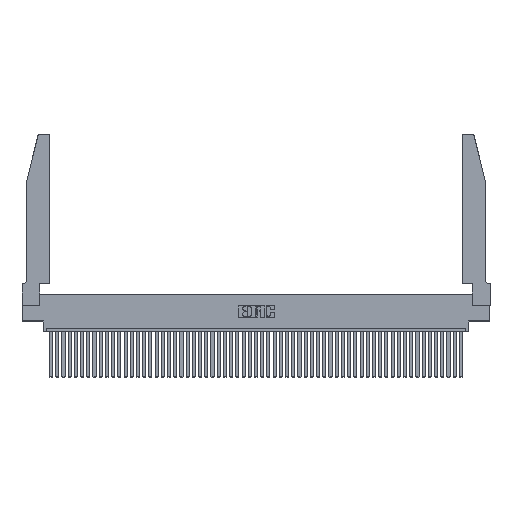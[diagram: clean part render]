
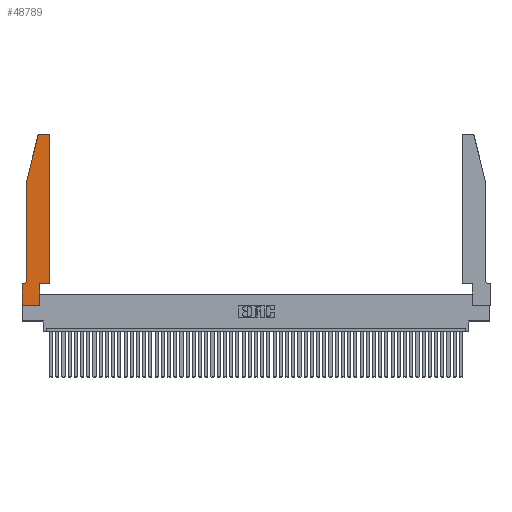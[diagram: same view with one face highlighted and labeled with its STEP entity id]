
A CAD part, top view. The second image highlights one B-rep face of the part: STEP entity #48789.
In plain terms, the highlighted planar face has unit normal (0, 0, 1).
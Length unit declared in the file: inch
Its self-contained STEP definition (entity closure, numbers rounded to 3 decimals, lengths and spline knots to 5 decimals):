
#66 = EDGE_CURVE ( 'NONE', #10024, #24313, #39739, .T. ) ;
#1700 = CARTESIAN_POINT ( 'NONE',  ( 0.2865, 0.35, 0.37 ) ) ;
#1920 = CARTESIAN_POINT ( 'NONE',  ( 0.2865, 0., 0.37 ) ) ;
#2434 = CARTESIAN_POINT ( 'NONE',  ( 0., 0., 0.37 ) ) ;
#2527 = VERTEX_POINT ( 'NONE', #1920 ) ;
#2875 = VECTOR ( 'NONE', #14905, 39.37008 ) ;
#3215 = EDGE_LOOP ( 'NONE', ( #14793, #34141, #24179, #48476, #18701, #36533, #26849, #27975, #34392, #27274, #50591, #46107 ) ) ;
#4255 = LINE ( 'NONE', #2434, #35532 ) ;
#4756 = VERTEX_POINT ( 'NONE', #42037 ) ;
#4902 = DIRECTION ( 'NONE',  ( 1., 0., 0. ) ) ;
#5426 = EDGE_CURVE ( 'NONE', #31566, #41945, #10612, .T. ) ;
#5642 = CARTESIAN_POINT ( 'NONE',  ( 0.284, 2.75, 0.37 ) ) ;
#7010 = CARTESIAN_POINT ( 'NONE',  ( 0.4205, 2.75, 0.37 ) ) ;
#7765 = DIRECTION ( 'NONE',  ( 0., 1., 0. ) ) ;
#8401 = LINE ( 'NONE', #18358, #28342 ) ;
#8618 = EDGE_CURVE ( 'NONE', #25354, #40194, #20551, .T. ) ;
#9263 = CARTESIAN_POINT ( 'NONE',  ( 0.0055, 0.42, 0.37 ) ) ;
#9737 = LINE ( 'NONE', #40828, #10432 ) ;
#10024 = VERTEX_POINT ( 'NONE', #45521 ) ;
#10281 = EDGE_CURVE ( 'NONE', #51760, #2527, #4255, .T. ) ;
#10432 = VECTOR ( 'NONE', #12880, 39.37008 ) ;
#10612 = LINE ( 'NONE', #22920, #39987 ) ;
#11596 = CARTESIAN_POINT ( 'NONE',  ( 0.4505, 0.35, 0.37 ) ) ;
#12880 = DIRECTION ( 'NONE',  ( -1., 0., 0. ) ) ;
#12923 = VECTOR ( 'NONE', #15116, 39.37008 ) ;
#13255 = DIRECTION ( 'NONE',  ( 0., 0., -1. ) ) ;
#13707 = VERTEX_POINT ( 'NONE', #30761 ) ;
#14534 = EDGE_CURVE ( 'NONE', #41945, #25354, #19542, .T. ) ;
#14793 = ORIENTED_EDGE ( 'NONE', *, *, #22210, .T. ) ;
#14905 = DIRECTION ( 'NONE',  ( -0.239, -0.971, 0. ) ) ;
#15116 = DIRECTION ( 'NONE',  ( 0., -1., 0. ) ) ;
#15321 = AXIS2_PLACEMENT_3D ( 'NONE', #49514, #17477, #21470 ) ;
#15543 = DIRECTION ( 'NONE',  ( 0., -1., 0. ) ) ;
#16575 = EDGE_CURVE ( 'NONE', #2527, #31566, #41148, .T. ) ;
#17477 = DIRECTION ( 'NONE',  ( 0., 0., 1. ) ) ;
#17835 = PLANE ( 'NONE',  #15321 ) ;
#18030 = CARTESIAN_POINT ( 'NONE',  ( 0., 0.35, 0.37 ) ) ;
#18358 = CARTESIAN_POINT ( 'NONE',  ( 0.2605, 2.75, 0.37 ) ) ;
#18701 = ORIENTED_EDGE ( 'NONE', *, *, #32629, .T. ) ;
#18705 = CARTESIAN_POINT ( 'NONE',  ( 0.0755, 2., 0.37 ) ) ;
#18867 = CARTESIAN_POINT ( 'NONE',  ( 0., 0., 0.37 ) ) ;
#19542 = LINE ( 'NONE', #11596, #29456 ) ;
#20551 = CIRCLE ( 'NONE', #43430, 0.03 ) ;
#20673 = CARTESIAN_POINT ( 'NONE',  ( 0.2865, 0.35, 0.37 ) ) ;
#20701 = CARTESIAN_POINT ( 'NONE',  ( 0.4205, 2.72, 0.37 ) ) ;
#21470 = DIRECTION ( 'NONE',  ( 1., 0., 0. ) ) ;
#22210 = EDGE_CURVE ( 'NONE', #40194, #28152, #8401, .T. ) ;
#22470 = DIRECTION ( 'NONE',  ( 1., 0., 0. ) ) ;
#22606 = CARTESIAN_POINT ( 'NONE',  ( 0.0755, 2., 0.37 ) ) ;
#22920 = CARTESIAN_POINT ( 'NONE',  ( 0.4505, 0.35, 0.37 ) ) ;
#22939 = LINE ( 'NONE', #22606, #12923 ) ;
#24179 = ORIENTED_EDGE ( 'NONE', *, *, #66, .T. ) ;
#24313 = VERTEX_POINT ( 'NONE', #28280 ) ;
#25354 = VERTEX_POINT ( 'NONE', #32321 ) ;
#26849 = ORIENTED_EDGE ( 'NONE', *, *, #44274, .T. ) ;
#26972 = DIRECTION ( 'NONE',  ( 1., 0., 0. ) ) ;
#27183 = FACE_OUTER_BOUND ( 'NONE', #3215, .T. ) ;
#27274 = ORIENTED_EDGE ( 'NONE', *, *, #5426, .T. ) ;
#27350 = DIRECTION ( 'NONE',  ( -1., 0., 0. ) ) ;
#27456 = CARTESIAN_POINT ( 'NONE',  ( 0., 0., 0.37 ) ) ;
#27975 = ORIENTED_EDGE ( 'NONE', *, *, #10281, .T. ) ;
#28152 = VERTEX_POINT ( 'NONE', #5642 ) ;
#28280 = CARTESIAN_POINT ( 'NONE',  ( 0.0755, 2., 0.37 ) ) ;
#28342 = VECTOR ( 'NONE', #27350, 39.37008 ) ;
#29274 = DIRECTION ( 'NONE',  ( -1., 0., 0. ) ) ;
#29456 = VECTOR ( 'NONE', #7765, 39.37008 ) ;
#30566 = VECTOR ( 'NONE', #44882, 39.37008 ) ;
#30761 = CARTESIAN_POINT ( 'NONE',  ( 0.0055, 0.35, 0.37 ) ) ;
#31566 = VERTEX_POINT ( 'NONE', #1700 ) ;
#31842 = CARTESIAN_POINT ( 'NONE',  ( 0.4505, 0.35, 0.37 ) ) ;
#32321 = CARTESIAN_POINT ( 'NONE',  ( 0.4505, 2.72, 0.37 ) ) ;
#32629 = EDGE_CURVE ( 'NONE', #4756, #13707, #36383, .T. ) ;
#33253 = AXIS2_PLACEMENT_3D ( 'NONE', #9263, #13255, #29274 ) ;
#34141 = ORIENTED_EDGE ( 'NONE', *, *, #34300, .T. ) ;
#34300 = EDGE_CURVE ( 'NONE', #28152, #10024, #47662, .T. ) ;
#34392 = ORIENTED_EDGE ( 'NONE', *, *, #16575, .T. ) ;
#34593 = VERTEX_POINT ( 'NONE', #18030 ) ;
#35532 = VECTOR ( 'NONE', #22470, 39.37008 ) ;
#36383 = CIRCLE ( 'NONE', #33253, 0.07 ) ;
#36533 = ORIENTED_EDGE ( 'NONE', *, *, #39883, .T. ) ;
#37733 = CARTESIAN_POINT ( 'NONE',  ( 0.284, 2.72, 0.37 ) ) ;
#39380 = VECTOR ( 'NONE', #15543, 39.37008 ) ;
#39534 = DIRECTION ( 'NONE',  ( 0., 0., 1. ) ) ;
#39739 = LINE ( 'NONE', #18705, #2875 ) ;
#39883 = EDGE_CURVE ( 'NONE', #13707, #34593, #9737, .T. ) ;
#39987 = VECTOR ( 'NONE', #26972, 39.37008 ) ;
#40194 = VERTEX_POINT ( 'NONE', #7010 ) ;
#40213 = DIRECTION ( 'NONE',  ( 0., 0., 1. ) ) ;
#40828 = CARTESIAN_POINT ( 'NONE',  ( 0.0755, 0.35, 0.37 ) ) ;
#41148 = LINE ( 'NONE', #20673, #30566 ) ;
#41945 = VERTEX_POINT ( 'NONE', #31842 ) ;
#42037 = CARTESIAN_POINT ( 'NONE',  ( 0.0755, 0.42, 0.37 ) ) ;
#43430 = AXIS2_PLACEMENT_3D ( 'NONE', #20701, #40213, #4902 ) ;
#44274 = EDGE_CURVE ( 'NONE', #34593, #51760, #48723, .T. ) ;
#44882 = DIRECTION ( 'NONE',  ( 0., 1., 0. ) ) ;
#45521 = CARTESIAN_POINT ( 'NONE',  ( 0.25487, 2.72718, 0.37 ) ) ;
#46107 = ORIENTED_EDGE ( 'NONE', *, *, #8618, .T. ) ;
#47055 = EDGE_CURVE ( 'NONE', #24313, #4756, #22939, .T. ) ;
#47662 = CIRCLE ( 'NONE', #49055, 0.03 ) ;
#48476 = ORIENTED_EDGE ( 'NONE', *, *, #47055, .T. ) ;
#48723 = LINE ( 'NONE', #27456, #39380 ) ;
#48789 = ADVANCED_FACE ( 'NONE', ( #27183 ), #17835, .T. ) ;
#49055 = AXIS2_PLACEMENT_3D ( 'NONE', #37733, #39534, #50936 ) ;
#49514 = CARTESIAN_POINT ( 'NONE',  ( 0., 0.35, 0.37 ) ) ;
#50591 = ORIENTED_EDGE ( 'NONE', *, *, #14534, .T. ) ;
#50936 = DIRECTION ( 'NONE',  ( 1., 0., 0. ) ) ;
#51760 = VERTEX_POINT ( 'NONE', #18867 ) ;
